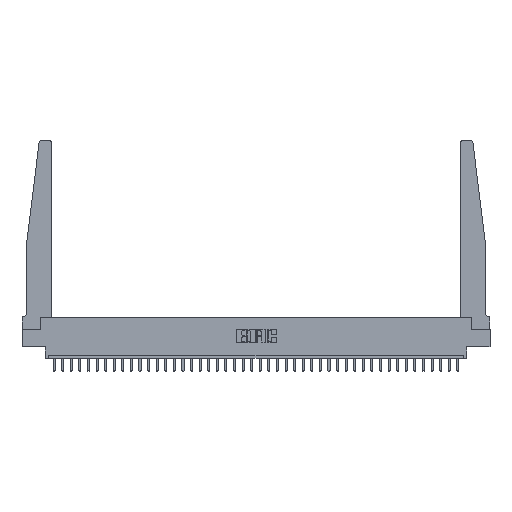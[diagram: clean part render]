
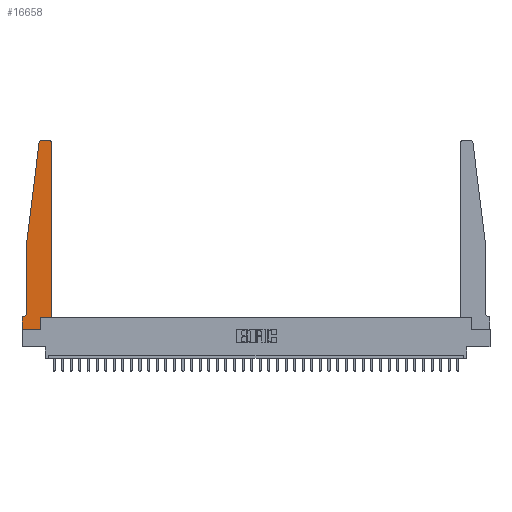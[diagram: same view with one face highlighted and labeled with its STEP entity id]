
A CAD part, top view. The second image highlights one B-rep face of the part: STEP entity #16658.
In plain terms, the highlighted planar face has unit normal (0, 0, 1).
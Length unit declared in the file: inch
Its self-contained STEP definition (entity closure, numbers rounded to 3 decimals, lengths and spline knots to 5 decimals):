
#78 = ORIENTED_EDGE ( 'NONE', *, *, #14989, .T. ) ;
#590 = DIRECTION ( 'NONE',  ( -1., 0., 0. ) ) ;
#1478 = EDGE_CURVE ( 'NONE', #29305, #11405, #13174, .T. ) ;
#1532 = DIRECTION ( 'NONE',  ( 0., -1., 0. ) ) ;
#1615 = VECTOR ( 'NONE', #29847, 39.37008 ) ;
#1650 = VECTOR ( 'NONE', #1532, 39.37008 ) ;
#1834 = EDGE_CURVE ( 'NONE', #30398, #28635, #11898, .T. ) ;
#1906 = DIRECTION ( 'NONE',  ( 0., -1., 0. ) ) ;
#2142 = DIRECTION ( 'NONE',  ( 0., 1., 0. ) ) ;
#2259 = DIRECTION ( 'NONE',  ( 0., 0., 1. ) ) ;
#2579 = AXIS2_PLACEMENT_3D ( 'NONE', #2985, #16256, #590 ) ;
#2985 = CARTESIAN_POINT ( 'NONE',  ( 0.015, 0.2375, 0.37 ) ) ;
#3276 = VERTEX_POINT ( 'NONE', #14748 ) ;
#3365 = VERTEX_POINT ( 'NONE', #23953 ) ;
#3373 = VECTOR ( 'NONE', #10913, 39.37008 ) ;
#4539 = LINE ( 'NONE', #17123, #24244 ) ;
#4871 = CARTESIAN_POINT ( 'NONE',  ( 0.395, 2.72, 0.37 ) ) ;
#4894 = CARTESIAN_POINT ( 'NONE',  ( 0.24675, 2.72367, 0.37 ) ) ;
#5107 = DIRECTION ( 'NONE',  ( 1., 0., 0. ) ) ;
#5177 = CARTESIAN_POINT ( 'NONE',  ( 0., 0.1875, 0.37 ) ) ;
#5741 = VECTOR ( 'NONE', #11309, 39.37008 ) ;
#6051 = CARTESIAN_POINT ( 'NONE',  ( 0.25, 2.75, 0.37 ) ) ;
#6217 = ORIENTED_EDGE ( 'NONE', *, *, #19328, .T. ) ;
#6352 = CARTESIAN_POINT ( 'NONE',  ( 0.065, 0.1875, 0.37 ) ) ;
#6363 = EDGE_CURVE ( 'NONE', #28635, #21455, #29076, .T. ) ;
#6530 = DIRECTION ( 'NONE',  ( 1., 0., 0. ) ) ;
#7298 = ORIENTED_EDGE ( 'NONE', *, *, #24891, .T. ) ;
#8020 = CARTESIAN_POINT ( 'NONE',  ( 0., 0.1875, 0.37 ) ) ;
#8707 = CARTESIAN_POINT ( 'NONE',  ( 0.2605, 0.18, 0.37 ) ) ;
#10045 = ORIENTED_EDGE ( 'NONE', *, *, #18333, .T. ) ;
#10109 = DIRECTION ( 'NONE',  ( 0., 1., 0. ) ) ;
#10913 = DIRECTION ( 'NONE',  ( -1., 0., 0. ) ) ;
#11091 = VERTEX_POINT ( 'NONE', #13891 ) ;
#11309 = DIRECTION ( 'NONE',  ( -0.122, -0.992, 0. ) ) ;
#11405 = VERTEX_POINT ( 'NONE', #29927 ) ;
#11898 = CIRCLE ( 'NONE', #2579, 0.05 ) ;
#12018 = DIRECTION ( 'NONE',  ( 0., 0., 1. ) ) ;
#12505 = ORIENTED_EDGE ( 'NONE', *, *, #12955, .T. ) ;
#12749 = CARTESIAN_POINT ( 'NONE',  ( 0.2605, 0.18, 0.37 ) ) ;
#12932 = EDGE_CURVE ( 'NONE', #18203, #3276, #32960, .T. ) ;
#12955 = EDGE_CURVE ( 'NONE', #31931, #3365, #13679, .T. ) ;
#13174 = LINE ( 'NONE', #32519, #5741 ) ;
#13436 = ORIENTED_EDGE ( 'NONE', *, *, #1834, .T. ) ;
#13679 = LINE ( 'NONE', #6051, #3373 ) ;
#13891 = CARTESIAN_POINT ( 'NONE',  ( 0., 0., 0.37 ) ) ;
#14492 = AXIS2_PLACEMENT_3D ( 'NONE', #4871, #2259, #5107 ) ;
#14748 = CARTESIAN_POINT ( 'NONE',  ( 0.425, 0.18, 0.37 ) ) ;
#14749 = VECTOR ( 'NONE', #6530, 39.37008 ) ;
#14927 = VERTEX_POINT ( 'NONE', #15064 ) ;
#14989 = EDGE_CURVE ( 'NONE', #14927, #31931, #30751, .T. ) ;
#15064 = CARTESIAN_POINT ( 'NONE',  ( 0.425, 2.72, 0.37 ) ) ;
#15495 = CARTESIAN_POINT ( 'NONE',  ( 0.015, 0.1875, 0.37 ) ) ;
#15616 = CIRCLE ( 'NONE', #30820, 0.03 ) ;
#16256 = DIRECTION ( 'NONE',  ( 0., 0., -1. ) ) ;
#16349 = ORIENTED_EDGE ( 'NONE', *, *, #1478, .T. ) ;
#16658 = ADVANCED_FACE ( 'NONE', ( #25306 ), #31471, .T. ) ;
#17123 = CARTESIAN_POINT ( 'NONE',  ( 0.065, 1.25, 0.37 ) ) ;
#17201 = CARTESIAN_POINT ( 'NONE',  ( 0., 0., 0.37 ) ) ;
#17744 = VERTEX_POINT ( 'NONE', #32102 ) ;
#17773 = AXIS2_PLACEMENT_3D ( 'NONE', #5177, #28811, #23526 ) ;
#17817 = CARTESIAN_POINT ( 'NONE',  ( 0.425, 0.18, 0.37 ) ) ;
#18203 = VERTEX_POINT ( 'NONE', #8707 ) ;
#18333 = EDGE_CURVE ( 'NONE', #3365, #29305, #15616, .T. ) ;
#19074 = EDGE_CURVE ( 'NONE', #11405, #30398, #4539, .T. ) ;
#19328 = EDGE_CURVE ( 'NONE', #21455, #11091, #31595, .T. ) ;
#19348 = ORIENTED_EDGE ( 'NONE', *, *, #6363, .T. ) ;
#21097 = ORIENTED_EDGE ( 'NONE', *, *, #12932, .T. ) ;
#21455 = VERTEX_POINT ( 'NONE', #8020 ) ;
#21841 = ORIENTED_EDGE ( 'NONE', *, *, #31829, .T. ) ;
#22429 = CARTESIAN_POINT ( 'NONE',  ( 0.27653, 2.72, 0.37 ) ) ;
#22720 = ORIENTED_EDGE ( 'NONE', *, *, #19074, .T. ) ;
#23163 = EDGE_LOOP ( 'NONE', ( #12505, #10045, #16349, #22720, #13436, #19348, #6217, #7298, #33005, #21097, #21841, #78 ) ) ;
#23371 = LINE ( 'NONE', #32983, #14749 ) ;
#23454 = CARTESIAN_POINT ( 'NONE',  ( 0.395, 2.75, 0.37 ) ) ;
#23526 = DIRECTION ( 'NONE',  ( 1., 0., 0. ) ) ;
#23555 = LINE ( 'NONE', #12749, #32223 ) ;
#23953 = CARTESIAN_POINT ( 'NONE',  ( 0.27653, 2.75, 0.37 ) ) ;
#24244 = VECTOR ( 'NONE', #1906, 39.37008 ) ;
#24293 = CARTESIAN_POINT ( 'NONE',  ( 0.425, 0.18, 0.37 ) ) ;
#24891 = EDGE_CURVE ( 'NONE', #11091, #17744, #23371, .T. ) ;
#25306 = FACE_OUTER_BOUND ( 'NONE', #23163, .T. ) ;
#25531 = LINE ( 'NONE', #17817, #30885 ) ;
#27813 = DIRECTION ( 'NONE',  ( 1., 0., 0. ) ) ;
#28635 = VERTEX_POINT ( 'NONE', #15495 ) ;
#28811 = DIRECTION ( 'NONE',  ( 0., 0., 1. ) ) ;
#29076 = LINE ( 'NONE', #6352, #1615 ) ;
#29305 = VERTEX_POINT ( 'NONE', #4894 ) ;
#29847 = DIRECTION ( 'NONE',  ( -1., 0., 0. ) ) ;
#29927 = CARTESIAN_POINT ( 'NONE',  ( 0.065, 1.25, 0.37 ) ) ;
#30183 = CARTESIAN_POINT ( 'NONE',  ( 0.065, 0.2375, 0.37 ) ) ;
#30398 = VERTEX_POINT ( 'NONE', #30183 ) ;
#30554 = EDGE_CURVE ( 'NONE', #17744, #18203, #23555, .T. ) ;
#30751 = CIRCLE ( 'NONE', #14492, 0.03 ) ;
#30820 = AXIS2_PLACEMENT_3D ( 'NONE', #22429, #12018, #27813 ) ;
#30885 = VECTOR ( 'NONE', #2142, 39.37008 ) ;
#31471 = PLANE ( 'NONE',  #17773 ) ;
#31595 = LINE ( 'NONE', #17201, #1650 ) ;
#31829 = EDGE_CURVE ( 'NONE', #3276, #14927, #25531, .T. ) ;
#31931 = VERTEX_POINT ( 'NONE', #23454 ) ;
#32102 = CARTESIAN_POINT ( 'NONE',  ( 0.2605, 0., 0.37 ) ) ;
#32122 = DIRECTION ( 'NONE',  ( 1., 0., 0. ) ) ;
#32144 = VECTOR ( 'NONE', #32122, 39.37008 ) ;
#32223 = VECTOR ( 'NONE', #10109, 39.37008 ) ;
#32519 = CARTESIAN_POINT ( 'NONE',  ( 0.065, 1.25, 0.37 ) ) ;
#32960 = LINE ( 'NONE', #24293, #32144 ) ;
#32983 = CARTESIAN_POINT ( 'NONE',  ( 0., 0., 0.37 ) ) ;
#33005 = ORIENTED_EDGE ( 'NONE', *, *, #30554, .T. ) ;
